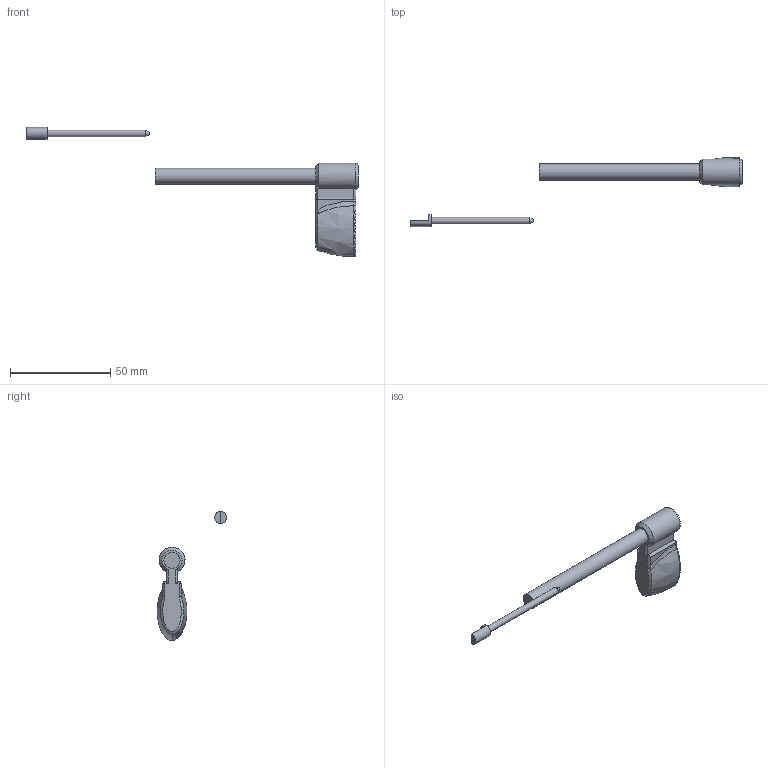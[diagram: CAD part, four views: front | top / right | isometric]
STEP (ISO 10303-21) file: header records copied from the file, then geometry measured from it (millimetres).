
FILE_DESCRIPTION(/* description */ (''),/* implementation_level */ '2;1');
FILE_NAME(/* author */ (''),/* organization */ (''),/* preprocessor_version */ 'ST-DEVELOPER v15.2',/* originating_system */ 'Autodesk Translator Framework v2.0.0.5431',/* authorisation */ '');
FILE_SCHEMA (('AUTOMOTIVE_DESIGN { 1 0 10303 214 3 1 1 }'));
Length unit declared in the file: centimetre
Products named in the file (1): (Unsaved)
Bounding box: 165.71 x 34.61 x 64.48 mm (x, y, z)
Volume: 13423.8 mm3; surface area: 6654.7 mm2
Topology: 3 solids, 3 shells, 187 faces, 491 edges, 319 vertices
Faces by surface type: plane 154, cylinder 15, bspline 11, cone 4, sphere 2, torus 1
Full cylindrical faces by diameter (mm): 3.254 x1, 6 x1, 8 x2
Entity records: 6600 total; most frequent: CARTESIAN_POINT 2131, ORIENTED_EDGE 960, DIRECTION 826, EDGE_CURVE 480, LINE 336, VECTOR 336, VERTEX_POINT 318, AXIS2_PLACEMENT_3D 245
